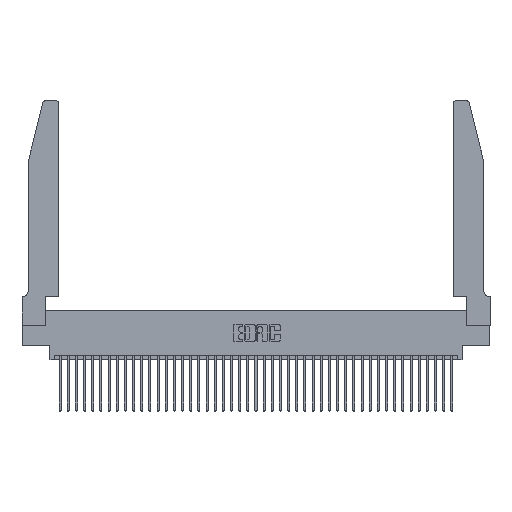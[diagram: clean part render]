
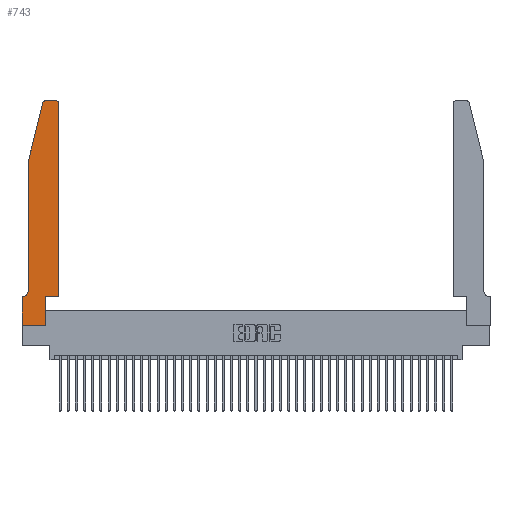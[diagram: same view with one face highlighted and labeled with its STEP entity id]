
A CAD part, top view. The second image highlights one B-rep face of the part: STEP entity #743.
In plain terms, the highlighted planar face has unit normal (0, 0, 1).
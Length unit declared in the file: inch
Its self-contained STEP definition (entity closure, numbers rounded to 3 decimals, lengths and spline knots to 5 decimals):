
#424 = CARTESIAN_POINT ( 'NONE',  ( 0., 0.35, 0.37 ) ) ;
#470 = ORIENTED_EDGE ( 'NONE', *, *, #22055, .T. ) ;
#743 = ADVANCED_FACE ( 'NONE', ( #17508 ), #2758, .T. ) ;
#1191 = CARTESIAN_POINT ( 'NONE',  ( 0.2605, 2.75, 0.37 ) ) ;
#2637 = DIRECTION ( 'NONE',  ( 0., 1., 0. ) ) ;
#2758 = PLANE ( 'NONE',  #6543 ) ;
#3009 = VECTOR ( 'NONE', #8004, 39.37008 ) ;
#3035 = EDGE_CURVE ( 'NONE', #28801, #40619, #28037, .T. ) ;
#3105 = VECTOR ( 'NONE', #15187, 39.37008 ) ;
#3520 = ORIENTED_EDGE ( 'NONE', *, *, #36867, .T. ) ;
#5128 = DIRECTION ( 'NONE',  ( 0., 0., 1. ) ) ;
#5397 = ORIENTED_EDGE ( 'NONE', *, *, #16427, .T. ) ;
#5791 = VERTEX_POINT ( 'NONE', #11686 ) ;
#6079 = DIRECTION ( 'NONE',  ( 1., 0., 0. ) ) ;
#6543 = AXIS2_PLACEMENT_3D ( 'NONE', #42014, #25889, #6079 ) ;
#6644 = ORIENTED_EDGE ( 'NONE', *, *, #28505, .T. ) ;
#6649 = CARTESIAN_POINT ( 'NONE',  ( 0.284, 2.75, 0.37 ) ) ;
#7037 = EDGE_CURVE ( 'NONE', #5791, #38537, #36997, .T. ) ;
#7890 = CARTESIAN_POINT ( 'NONE',  ( 0.0755, 0.42, 0.37 ) ) ;
#8004 = DIRECTION ( 'NONE',  ( -1., 0., 0. ) ) ;
#8387 = CARTESIAN_POINT ( 'NONE',  ( 0.0755, 2., 0.37 ) ) ;
#8416 = VECTOR ( 'NONE', #30857, 39.37008 ) ;
#8451 = CARTESIAN_POINT ( 'NONE',  ( 0.4505, 0.35, 0.37 ) ) ;
#9216 = CARTESIAN_POINT ( 'NONE',  ( 0.0755, 2., 0.37 ) ) ;
#9605 = EDGE_CURVE ( 'NONE', #33386, #33352, #35290, .T. ) ;
#9750 = ORIENTED_EDGE ( 'NONE', *, *, #22794, .T. ) ;
#10200 = VECTOR ( 'NONE', #14860, 39.37008 ) ;
#10365 = VECTOR ( 'NONE', #25001, 39.37008 ) ;
#10535 = ORIENTED_EDGE ( 'NONE', *, *, #7037, .T. ) ;
#10596 = CARTESIAN_POINT ( 'NONE',  ( 0.4505, 0.35, 0.37 ) ) ;
#11424 = ORIENTED_EDGE ( 'NONE', *, *, #27908, .T. ) ;
#11455 = DIRECTION ( 'NONE',  ( 0., -1., 0. ) ) ;
#11686 = CARTESIAN_POINT ( 'NONE',  ( 0.2865, 0., 0.37 ) ) ;
#12292 = LINE ( 'NONE', #8387, #37344 ) ;
#12337 = LINE ( 'NONE', #10596, #37391 ) ;
#12843 = ORIENTED_EDGE ( 'NONE', *, *, #9605, .T. ) ;
#13032 = AXIS2_PLACEMENT_3D ( 'NONE', #15929, #38683, #19274 ) ;
#13587 = DIRECTION ( 'NONE',  ( 0., -1., 0. ) ) ;
#13721 = CARTESIAN_POINT ( 'NONE',  ( 0., 0., 0.37 ) ) ;
#13964 = DIRECTION ( 'NONE',  ( 1., 0., 0. ) ) ;
#14272 = CARTESIAN_POINT ( 'NONE',  ( 0.4505, 2.72, 0.37 ) ) ;
#14860 = DIRECTION ( 'NONE',  ( -0.239, -0.971, 0. ) ) ;
#15187 = DIRECTION ( 'NONE',  ( 0., 1., 0. ) ) ;
#15487 = ORIENTED_EDGE ( 'NONE', *, *, #3035, .T. ) ;
#15780 = VERTEX_POINT ( 'NONE', #8451 ) ;
#15929 = CARTESIAN_POINT ( 'NONE',  ( 0.284, 2.72, 0.37 ) ) ;
#16163 = DIRECTION ( 'NONE',  ( 0., 0., -1. ) ) ;
#16427 = EDGE_CURVE ( 'NONE', #15780, #42013, #40115, .T. ) ;
#16571 = CARTESIAN_POINT ( 'NONE',  ( 0.0055, 0.35, 0.37 ) ) ;
#16905 = ORIENTED_EDGE ( 'NONE', *, *, #40089, .T. ) ;
#17342 = CARTESIAN_POINT ( 'NONE',  ( 0.0755, 0.35, 0.37 ) ) ;
#17508 = FACE_OUTER_BOUND ( 'NONE', #21952, .T. ) ;
#17601 = EDGE_CURVE ( 'NONE', #18816, #34214, #35694, .T. ) ;
#18407 = EDGE_CURVE ( 'NONE', #40619, #33386, #30670, .T. ) ;
#18816 = VERTEX_POINT ( 'NONE', #7890 ) ;
#19203 = LINE ( 'NONE', #31542, #10365 ) ;
#19274 = DIRECTION ( 'NONE',  ( 1., 0., 0. ) ) ;
#19554 = CARTESIAN_POINT ( 'NONE',  ( 0.25487, 2.72718, 0.37 ) ) ;
#19661 = CARTESIAN_POINT ( 'NONE',  ( 0.4205, 2.75, 0.37 ) ) ;
#20254 = VERTEX_POINT ( 'NONE', #25132 ) ;
#21952 = EDGE_LOOP ( 'NONE', ( #15487, #23205, #12843, #9750, #26744, #470, #3520, #11424, #10535, #16905, #5397, #6644 ) ) ;
#22055 = EDGE_CURVE ( 'NONE', #34214, #37709, #30364, .T. ) ;
#22794 = EDGE_CURVE ( 'NONE', #33352, #18816, #12292, .T. ) ;
#23205 = ORIENTED_EDGE ( 'NONE', *, *, #18407, .T. ) ;
#24627 = CARTESIAN_POINT ( 'NONE',  ( 0.2865, 0.35, 0.37 ) ) ;
#24945 = CARTESIAN_POINT ( 'NONE',  ( 0.4205, 2.72, 0.37 ) ) ;
#25001 = DIRECTION ( 'NONE',  ( 1., 0., 0. ) ) ;
#25132 = CARTESIAN_POINT ( 'NONE',  ( 0., 0., 0.37 ) ) ;
#25260 = LINE ( 'NONE', #13721, #41430 ) ;
#25616 = CARTESIAN_POINT ( 'NONE',  ( 0.4505, 0.35, 0.37 ) ) ;
#25889 = DIRECTION ( 'NONE',  ( 0., 0., 1. ) ) ;
#26744 = ORIENTED_EDGE ( 'NONE', *, *, #17601, .T. ) ;
#27908 = EDGE_CURVE ( 'NONE', #20254, #5791, #19203, .T. ) ;
#28037 = LINE ( 'NONE', #1191, #8416 ) ;
#28214 = DIRECTION ( 'NONE',  ( 1., 0., 0. ) ) ;
#28505 = EDGE_CURVE ( 'NONE', #42013, #28801, #31403, .T. ) ;
#28801 = VERTEX_POINT ( 'NONE', #19661 ) ;
#30364 = LINE ( 'NONE', #17342, #3009 ) ;
#30670 = CIRCLE ( 'NONE', #13032, 0.03 ) ;
#30857 = DIRECTION ( 'NONE',  ( -1., 0., 0. ) ) ;
#30878 = AXIS2_PLACEMENT_3D ( 'NONE', #35669, #16163, #38922 ) ;
#31403 = CIRCLE ( 'NONE', #32374, 0.03 ) ;
#31525 = CARTESIAN_POINT ( 'NONE',  ( 0.2865, 0.35, 0.37 ) ) ;
#31542 = CARTESIAN_POINT ( 'NONE',  ( 0., 0., 0.37 ) ) ;
#31568 = VECTOR ( 'NONE', #2637, 39.37008 ) ;
#32374 = AXIS2_PLACEMENT_3D ( 'NONE', #24945, #5128, #28214 ) ;
#33352 = VERTEX_POINT ( 'NONE', #9216 ) ;
#33386 = VERTEX_POINT ( 'NONE', #19554 ) ;
#34214 = VERTEX_POINT ( 'NONE', #16571 ) ;
#34439 = CARTESIAN_POINT ( 'NONE',  ( 0.0755, 2., 0.37 ) ) ;
#35290 = LINE ( 'NONE', #34439, #10200 ) ;
#35669 = CARTESIAN_POINT ( 'NONE',  ( 0.0055, 0.42, 0.37 ) ) ;
#35694 = CIRCLE ( 'NONE', #30878, 0.07 ) ;
#36867 = EDGE_CURVE ( 'NONE', #37709, #20254, #25260, .T. ) ;
#36997 = LINE ( 'NONE', #31525, #3105 ) ;
#37344 = VECTOR ( 'NONE', #11455, 39.37008 ) ;
#37391 = VECTOR ( 'NONE', #13964, 39.37008 ) ;
#37709 = VERTEX_POINT ( 'NONE', #424 ) ;
#38537 = VERTEX_POINT ( 'NONE', #24627 ) ;
#38683 = DIRECTION ( 'NONE',  ( 0., 0., 1. ) ) ;
#38922 = DIRECTION ( 'NONE',  ( -1., 0., 0. ) ) ;
#40089 = EDGE_CURVE ( 'NONE', #38537, #15780, #12337, .T. ) ;
#40115 = LINE ( 'NONE', #25616, #31568 ) ;
#40619 = VERTEX_POINT ( 'NONE', #6649 ) ;
#41430 = VECTOR ( 'NONE', #13587, 39.37008 ) ;
#42013 = VERTEX_POINT ( 'NONE', #14272 ) ;
#42014 = CARTESIAN_POINT ( 'NONE',  ( 0., 0.35, 0.37 ) ) ;
